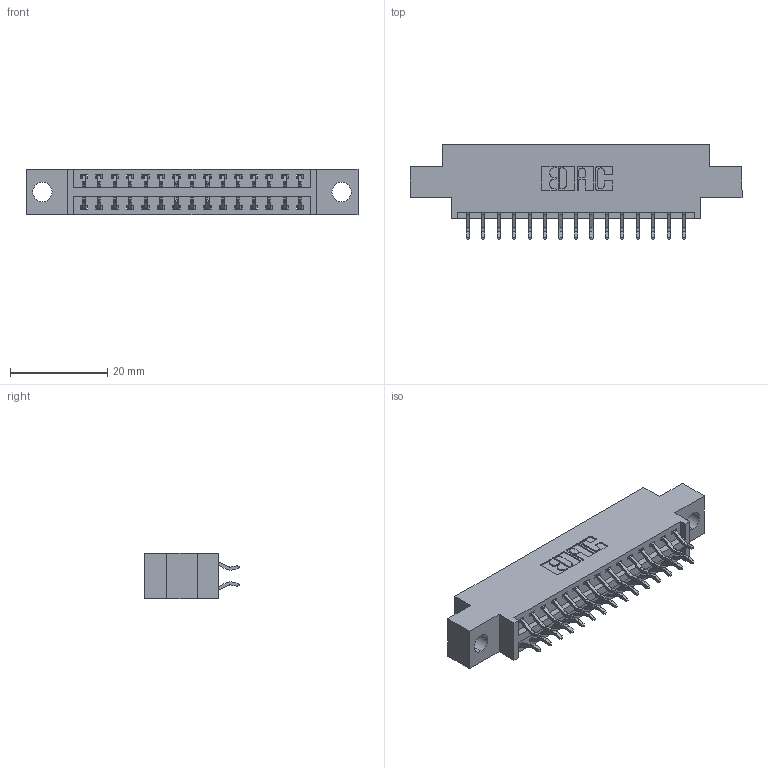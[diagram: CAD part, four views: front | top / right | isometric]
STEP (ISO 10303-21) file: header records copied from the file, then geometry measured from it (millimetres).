
FILE_DESCRIPTION (( 'STEP AP203' ), '1' );
FILE_NAME ('396-030-556-804.STEP', '2019-11-01T19:49:44', ( '' ), ( '' ), 'SwSTEP 2.0', 'SolidWorks 2016', '' );
FILE_SCHEMA (( 'CONFIG_CONTROL_DESIGN' ));
Length unit declared in the file: inch
Products named in the file (3): 396-030-556-804; 346 Part_0.170 Offset - 0.156 Dia-TH; 345-292-001_556 Tail
Assembly tree (31 placements, depth 2):
  396-030-556-804
    346 Part_0.170 Offset - 0.156 Dia-TH
    345-292-001_556 Tail  x30
Bounding box: 68.2 x 19.57 x 9.4 mm (x, y, z)
Volume: 6196.9 mm3; surface area: 8058.8 mm2
Topology: 31 solids, 31 shells, 1866 faces, 5531 edges, 3646 vertices
Faces by surface type: plane 1250, cylinder 616
Entity records: 13779 total; most frequent: CARTESIAN_POINT 2324, ORIENTED_EDGE 2246, DIRECTION 2087, EDGE_CURVE 1123, LINE 923, VECTOR 923, VERTEX_POINT 746, AXIS2_PLACEMENT_3D 582
